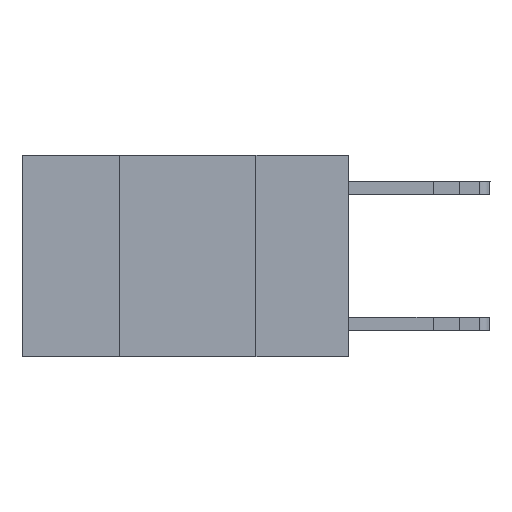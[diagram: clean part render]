
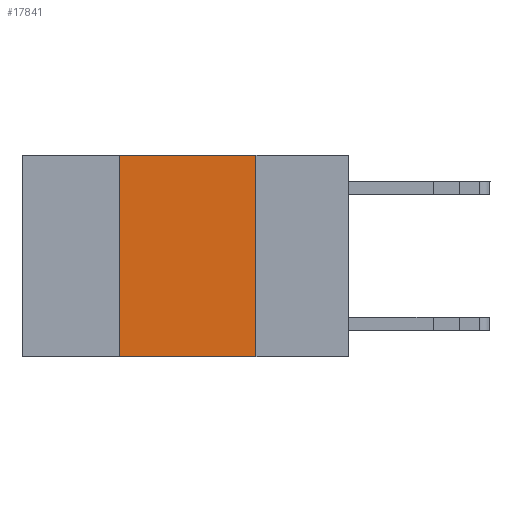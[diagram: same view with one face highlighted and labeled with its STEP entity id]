
A CAD part, left-side view. The second image highlights one B-rep face of the part: STEP entity #17841.
In plain terms, the highlighted planar face has unit normal (-1, 0, 0).
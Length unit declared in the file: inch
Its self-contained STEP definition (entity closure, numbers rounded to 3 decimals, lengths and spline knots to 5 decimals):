
#467 = VECTOR ( 'NONE', #1781, 39.37008 ) ;
#1781 = DIRECTION ( 'NONE',  ( 0., -1., 0. ) ) ;
#2576 = PLANE ( 'NONE',  #7315 ) ;
#3452 = LINE ( 'NONE', #6536, #19445 ) ;
#3697 = VECTOR ( 'NONE', #4151, 39.37008 ) ;
#4151 = DIRECTION ( 'NONE',  ( 0., 0., 1. ) ) ;
#6536 = CARTESIAN_POINT ( 'NONE',  ( 0., 0.17, 0. ) ) ;
#6662 = DIRECTION ( 'NONE',  ( 0., 0., -1. ) ) ;
#7315 = AXIS2_PLACEMENT_3D ( 'NONE', #23313, #16025, #23690 ) ;
#7486 = LINE ( 'NONE', #24528, #467 ) ;
#7594 = CARTESIAN_POINT ( 'NONE',  ( 0., 0.42, 0. ) ) ;
#10668 = CARTESIAN_POINT ( 'NONE',  ( 0., 0.6, 0. ) ) ;
#10788 = DIRECTION ( 'NONE',  ( 0., -1., 0. ) ) ;
#11101 = VERTEX_POINT ( 'NONE', #12319 ) ;
#11532 = EDGE_CURVE ( 'NONE', #14513, #11101, #18026, .T. ) ;
#11846 = ORIENTED_EDGE ( 'NONE', *, *, #21055, .F. ) ;
#11863 = CARTESIAN_POINT ( 'NONE',  ( 0., 0.42, -0.37 ) ) ;
#12068 = CARTESIAN_POINT ( 'NONE',  ( 0., 0.17, -0.37 ) ) ;
#12319 = CARTESIAN_POINT ( 'NONE',  ( 0., 0.17, 0. ) ) ;
#14513 = VERTEX_POINT ( 'NONE', #15119 ) ;
#15119 = CARTESIAN_POINT ( 'NONE',  ( 0., 0.42, 0. ) ) ;
#15285 = EDGE_CURVE ( 'NONE', #11101, #16868, #3452, .T. ) ;
#15534 = VERTEX_POINT ( 'NONE', #11863 ) ;
#15668 = FACE_OUTER_BOUND ( 'NONE', #15881, .T. ) ;
#15881 = EDGE_LOOP ( 'NONE', ( #18879, #20967, #11846, #23386 ) ) ;
#16025 = DIRECTION ( 'NONE',  ( 1., 0., 0. ) ) ;
#16868 = VERTEX_POINT ( 'NONE', #12068 ) ;
#17737 = VECTOR ( 'NONE', #10788, 39.37008 ) ;
#17841 = ADVANCED_FACE ( 'NONE', ( #15668 ), #2576, .F. ) ;
#18026 = LINE ( 'NONE', #10668, #17737 ) ;
#18879 = ORIENTED_EDGE ( 'NONE', *, *, #15285, .F. ) ;
#19445 = VECTOR ( 'NONE', #6662, 39.37008 ) ;
#20059 = EDGE_CURVE ( 'NONE', #15534, #16868, #7486, .T. ) ;
#20967 = ORIENTED_EDGE ( 'NONE', *, *, #11532, .F. ) ;
#21055 = EDGE_CURVE ( 'NONE', #15534, #14513, #24649, .T. ) ;
#23313 = CARTESIAN_POINT ( 'NONE',  ( 0., 0.6, 0. ) ) ;
#23386 = ORIENTED_EDGE ( 'NONE', *, *, #20059, .T. ) ;
#23690 = DIRECTION ( 'NONE',  ( 0., 0., -1. ) ) ;
#24528 = CARTESIAN_POINT ( 'NONE',  ( 0., 0.6, -0.37 ) ) ;
#24649 = LINE ( 'NONE', #7594, #3697 ) ;
